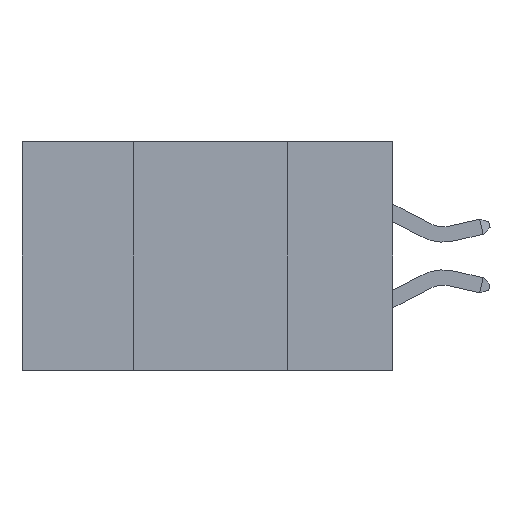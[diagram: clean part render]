
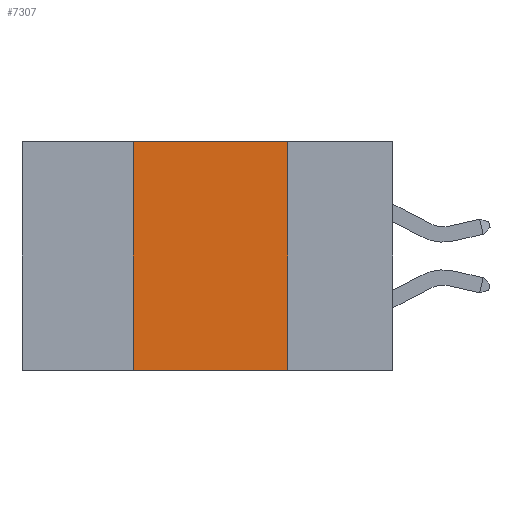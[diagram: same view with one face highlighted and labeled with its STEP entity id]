
A CAD part, left-side view. The second image highlights one B-rep face of the part: STEP entity #7307.
In plain terms, the highlighted planar face has unit normal (-1, 0, 0).
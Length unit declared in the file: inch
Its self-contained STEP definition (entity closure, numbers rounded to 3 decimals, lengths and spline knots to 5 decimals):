
#138 = AXIS2_PLACEMENT_3D ( 'NONE', #10218, #6255, #15101 ) ;
#306 = EDGE_CURVE ( 'NONE', #15293, #5209, #14853, .T. ) ;
#3451 = EDGE_LOOP ( 'NONE', ( #14248, #4298, #4747, #12967 ) ) ;
#3458 = CARTESIAN_POINT ( 'NONE',  ( 0., 0.42, -0.37 ) ) ;
#4298 = ORIENTED_EDGE ( 'NONE', *, *, #11330, .F. ) ;
#4747 = ORIENTED_EDGE ( 'NONE', *, *, #9668, .F. ) ;
#5014 = VERTEX_POINT ( 'NONE', #8971 ) ;
#5107 = VECTOR ( 'NONE', #13127, 39.37008 ) ;
#5209 = VERTEX_POINT ( 'NONE', #15475 ) ;
#5278 = FACE_OUTER_BOUND ( 'NONE', #3451, .T. ) ;
#5406 = LINE ( 'NONE', #14511, #11982 ) ;
#5644 = VECTOR ( 'NONE', #16631, 39.37008 ) ;
#5934 = DIRECTION ( 'NONE',  ( 0., -1., 0. ) ) ;
#6255 = DIRECTION ( 'NONE',  ( 1., 0., 0. ) ) ;
#6977 = DIRECTION ( 'NONE',  ( 0., -1., 0. ) ) ;
#7307 = ADVANCED_FACE ( 'NONE', ( #5278 ), #12696, .F. ) ;
#8971 = CARTESIAN_POINT ( 'NONE',  ( 0., 0.17, 0. ) ) ;
#9668 = EDGE_CURVE ( 'NONE', #15293, #13338, #15386, .T. ) ;
#10218 = CARTESIAN_POINT ( 'NONE',  ( 0., 0.6, 0. ) ) ;
#11288 = VECTOR ( 'NONE', #5934, 39.37008 ) ;
#11330 = EDGE_CURVE ( 'NONE', #13338, #5014, #5406, .T. ) ;
#11982 = VECTOR ( 'NONE', #6977, 39.37008 ) ;
#11993 = CARTESIAN_POINT ( 'NONE',  ( 0., 0.17, 0. ) ) ;
#12117 = LINE ( 'NONE', #11993, #5107 ) ;
#12696 = PLANE ( 'NONE',  #138 ) ;
#12883 = EDGE_CURVE ( 'NONE', #5014, #5209, #12117, .T. ) ;
#12967 = ORIENTED_EDGE ( 'NONE', *, *, #306, .T. ) ;
#13127 = DIRECTION ( 'NONE',  ( 0., 0., -1. ) ) ;
#13338 = VERTEX_POINT ( 'NONE', #16382 ) ;
#14248 = ORIENTED_EDGE ( 'NONE', *, *, #12883, .F. ) ;
#14511 = CARTESIAN_POINT ( 'NONE',  ( 0., 0.6, 0. ) ) ;
#14681 = CARTESIAN_POINT ( 'NONE',  ( 0., 0.6, -0.37 ) ) ;
#14853 = LINE ( 'NONE', #14681, #11288 ) ;
#15101 = DIRECTION ( 'NONE',  ( 0., 0., -1. ) ) ;
#15293 = VERTEX_POINT ( 'NONE', #3458 ) ;
#15369 = CARTESIAN_POINT ( 'NONE',  ( 0., 0.42, 0. ) ) ;
#15386 = LINE ( 'NONE', #15369, #5644 ) ;
#15475 = CARTESIAN_POINT ( 'NONE',  ( 0., 0.17, -0.37 ) ) ;
#16382 = CARTESIAN_POINT ( 'NONE',  ( 0., 0.42, 0. ) ) ;
#16631 = DIRECTION ( 'NONE',  ( 0., 0., 1. ) ) ;
